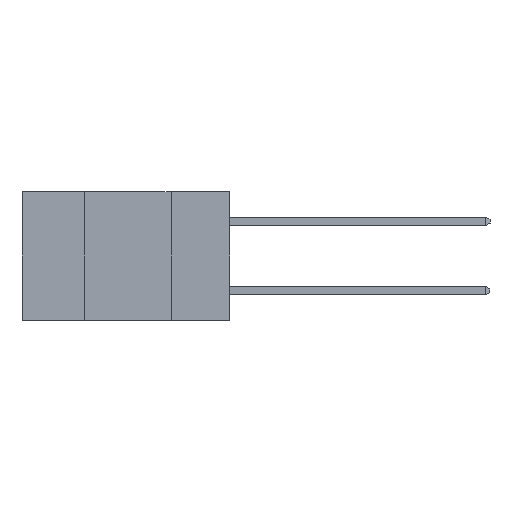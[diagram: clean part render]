
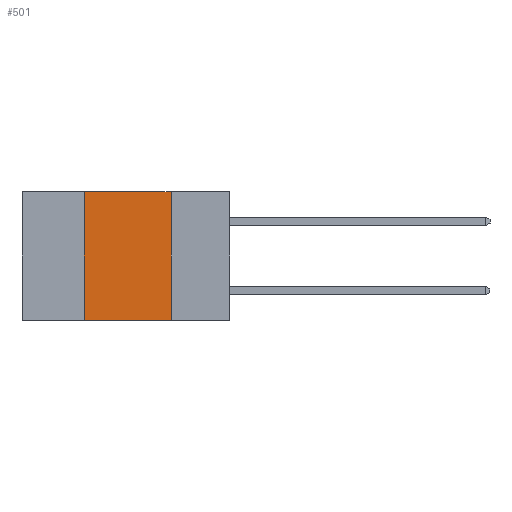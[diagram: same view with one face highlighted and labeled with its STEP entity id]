
A CAD part, left-side view. The second image highlights one B-rep face of the part: STEP entity #501.
In plain terms, the highlighted planar face has unit normal (-1, 0, 0).
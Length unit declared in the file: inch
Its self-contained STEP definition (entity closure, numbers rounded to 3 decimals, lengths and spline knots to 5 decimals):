
#214 = DIRECTION ( 'NONE',  ( 0., -1., 0. ) ) ;
#253 = LINE ( 'NONE', #1952, #7057 ) ;
#501 = ADVANCED_FACE ( 'NONE', ( #4797 ), #5767, .F. ) ;
#881 = ORIENTED_EDGE ( 'NONE', *, *, #1017, .F. ) ;
#1017 = EDGE_CURVE ( 'NONE', #1545, #6277, #253, .T. ) ;
#1335 = ORIENTED_EDGE ( 'NONE', *, *, #14184, .F. ) ;
#1545 = VERTEX_POINT ( 'NONE', #2403 ) ;
#1819 = DIRECTION ( 'NONE',  ( 0., 0., -1. ) ) ;
#1952 = CARTESIAN_POINT ( 'NONE',  ( 0., 0.17, 0. ) ) ;
#2118 = ORIENTED_EDGE ( 'NONE', *, *, #10879, .F. ) ;
#2403 = CARTESIAN_POINT ( 'NONE',  ( 0., 0.17, 0. ) ) ;
#2437 = LINE ( 'NONE', #13116, #9149 ) ;
#3598 = DIRECTION ( 'NONE',  ( 0., -1., 0. ) ) ;
#4797 = FACE_OUTER_BOUND ( 'NONE', #14212, .T. ) ;
#5748 = DIRECTION ( 'NONE',  ( 0., 0., -1. ) ) ;
#5758 = ORIENTED_EDGE ( 'NONE', *, *, #12929, .T. ) ;
#5765 = DIRECTION ( 'NONE',  ( 1., 0., 0. ) ) ;
#5767 = PLANE ( 'NONE',  #10206 ) ;
#5880 = CARTESIAN_POINT ( 'NONE',  ( 0., 0.6, 0. ) ) ;
#6277 = VERTEX_POINT ( 'NONE', #14130 ) ;
#6293 = LINE ( 'NONE', #15413, #12916 ) ;
#7057 = VECTOR ( 'NONE', #1819, 39.37008 ) ;
#7560 = CARTESIAN_POINT ( 'NONE',  ( 0., 0.6, -0.37 ) ) ;
#7969 = CARTESIAN_POINT ( 'NONE',  ( 0., 0.42, 0. ) ) ;
#8195 = DIRECTION ( 'NONE',  ( 0., 0., 1. ) ) ;
#9149 = VECTOR ( 'NONE', #214, 39.37008 ) ;
#10206 = AXIS2_PLACEMENT_3D ( 'NONE', #5880, #5765, #5748 ) ;
#10549 = VECTOR ( 'NONE', #3598, 39.37008 ) ;
#10690 = VERTEX_POINT ( 'NONE', #7969 ) ;
#10879 = EDGE_CURVE ( 'NONE', #10690, #1545, #2437, .T. ) ;
#12916 = VECTOR ( 'NONE', #8195, 39.37008 ) ;
#12929 = EDGE_CURVE ( 'NONE', #14639, #6277, #13725, .T. ) ;
#13116 = CARTESIAN_POINT ( 'NONE',  ( 0., 0.6, 0. ) ) ;
#13725 = LINE ( 'NONE', #7560, #10549 ) ;
#14130 = CARTESIAN_POINT ( 'NONE',  ( 0., 0.17, -0.37 ) ) ;
#14184 = EDGE_CURVE ( 'NONE', #14639, #10690, #6293, .T. ) ;
#14212 = EDGE_LOOP ( 'NONE', ( #881, #2118, #1335, #5758 ) ) ;
#14639 = VERTEX_POINT ( 'NONE', #15010 ) ;
#15010 = CARTESIAN_POINT ( 'NONE',  ( 0., 0.42, -0.37 ) ) ;
#15413 = CARTESIAN_POINT ( 'NONE',  ( 0., 0.42, 0. ) ) ;
